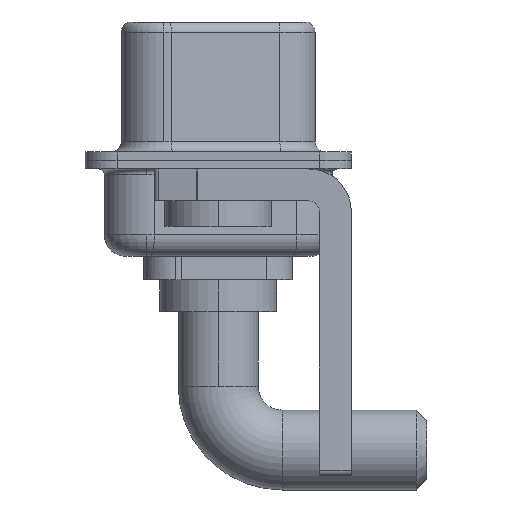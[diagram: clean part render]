
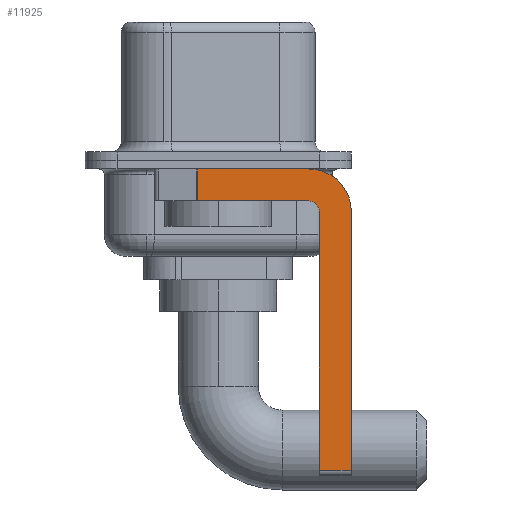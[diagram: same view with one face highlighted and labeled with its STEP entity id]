
A CAD part, left-side view. The second image highlights one B-rep face of the part: STEP entity #11925.
In plain terms, the highlighted planar face has unit normal (-1, 0, 0).
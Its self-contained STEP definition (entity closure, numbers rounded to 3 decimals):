
#54 = LINE ( 'NONE', #5189, #10885 ) ;
#91 = CARTESIAN_POINT ( 'NONE',  ( -2.9, -6.25, -2.4 ) ) ;
#367 = DIRECTION ( 'NONE',  ( 0., -1., 0. ) ) ;
#451 = DIRECTION ( 'NONE',  ( 1., 0., 0. ) ) ;
#596 = VECTOR ( 'NONE', #11595, 1000. ) ;
#710 = VERTEX_POINT ( 'NONE', #9211 ) ;
#754 = VERTEX_POINT ( 'NONE', #5790 ) ;
#1025 = EDGE_CURVE ( 'NONE', #7163, #14038, #7813, .T. ) ;
#1320 = VECTOR ( 'NONE', #367, 1000. ) ;
#1336 = VECTOR ( 'NONE', #6732, 1000. ) ;
#1689 = CARTESIAN_POINT ( 'NONE',  ( -2.9, -4.75, -2.4 ) ) ;
#1849 = ORIENTED_EDGE ( 'NONE', *, *, #5173, .T. ) ;
#1904 = CARTESIAN_POINT ( 'NONE',  ( -2.9, 0.978, -0.4 ) ) ;
#2360 = VECTOR ( 'NONE', #4473, 1000. ) ;
#2472 = EDGE_CURVE ( 'NONE', #4722, #754, #10742, .T. ) ;
#2613 = CARTESIAN_POINT ( 'NONE',  ( -2.9, -4.25, -1.9 ) ) ;
#2647 = CARTESIAN_POINT ( 'NONE',  ( -2.9, 0.978, -1.9 ) ) ;
#2786 = ORIENTED_EDGE ( 'NONE', *, *, #13909, .F. ) ;
#3198 = CARTESIAN_POINT ( 'NONE',  ( -2.9, -4.75, -14.55 ) ) ;
#3556 = CIRCLE ( 'NONE', #6793, 2. ) ;
#3600 = DIRECTION ( 'NONE',  ( -1., 0., 0. ) ) ;
#4473 = DIRECTION ( 'NONE',  ( 0., 0., -1. ) ) ;
#4722 = VERTEX_POINT ( 'NONE', #1904 ) ;
#5173 = EDGE_CURVE ( 'NONE', #16331, #710, #11849, .T. ) ;
#5189 = CARTESIAN_POINT ( 'NONE',  ( -2.9, 3., -0.4 ) ) ;
#5223 = DIRECTION ( 'NONE',  ( 0., 1., 0. ) ) ;
#5396 = LINE ( 'NONE', #6495, #596 ) ;
#5439 = DIRECTION ( 'NONE',  ( 0., 0., -1. ) ) ;
#5602 = EDGE_CURVE ( 'NONE', #6083, #710, #14275, .T. ) ;
#5678 = CARTESIAN_POINT ( 'NONE',  ( -2.9, -4.25, -1.9 ) ) ;
#5790 = CARTESIAN_POINT ( 'NONE',  ( -2.9, 0.978, -1.9 ) ) ;
#6025 = AXIS2_PLACEMENT_3D ( 'NONE', #15941, #13123, #5439 ) ;
#6038 = ORIENTED_EDGE ( 'NONE', *, *, #6094, .F. ) ;
#6083 = VERTEX_POINT ( 'NONE', #91 ) ;
#6094 = EDGE_CURVE ( 'NONE', #14038, #754, #11581, .T. ) ;
#6495 = CARTESIAN_POINT ( 'NONE',  ( -2.9, -4.75, -14.8 ) ) ;
#6732 = DIRECTION ( 'NONE',  ( 0., 0., -1. ) ) ;
#6793 = AXIS2_PLACEMENT_3D ( 'NONE', #11931, #451, #14552 ) ;
#7163 = VERTEX_POINT ( 'NONE', #1689 ) ;
#7592 = ORIENTED_EDGE ( 'NONE', *, *, #8351, .F. ) ;
#7813 = CIRCLE ( 'NONE', #14800, 0.5 ) ;
#8167 = CARTESIAN_POINT ( 'NONE',  ( -2.9, -4.25, -14.55 ) ) ;
#8351 = EDGE_CURVE ( 'NONE', #16331, #7163, #5396, .T. ) ;
#8364 = PLANE ( 'NONE',  #6025 ) ;
#8533 = VERTEX_POINT ( 'NONE', #12171 ) ;
#9000 = EDGE_LOOP ( 'NONE', ( #2786, #15157, #6038, #12072, #7592, #1849, #15802, #12744 ) ) ;
#9030 = CARTESIAN_POINT ( 'NONE',  ( -2.9, -4.25, -2.4 ) ) ;
#9211 = CARTESIAN_POINT ( 'NONE',  ( -2.9, -6.25, -14.55 ) ) ;
#9973 = EDGE_CURVE ( 'NONE', #8533, #6083, #3556, .T. ) ;
#10038 = DIRECTION ( 'NONE',  ( 0., 0., 1. ) ) ;
#10424 = CARTESIAN_POINT ( 'NONE',  ( -2.9, -6.25, -2.4 ) ) ;
#10742 = LINE ( 'NONE', #2647, #2360 ) ;
#10885 = VECTOR ( 'NONE', #15432, 1000. ) ;
#10986 = VECTOR ( 'NONE', #5223, 1000. ) ;
#11581 = LINE ( 'NONE', #2613, #10986 ) ;
#11595 = DIRECTION ( 'NONE',  ( 0., 0., 1. ) ) ;
#11849 = LINE ( 'NONE', #8167, #1320 ) ;
#11925 = ADVANCED_FACE ( 'NONE', ( #14399 ), #8364, .F. ) ;
#11931 = CARTESIAN_POINT ( 'NONE',  ( -2.9, -4.25, -2.4 ) ) ;
#12072 = ORIENTED_EDGE ( 'NONE', *, *, #1025, .F. ) ;
#12171 = CARTESIAN_POINT ( 'NONE',  ( -2.9, -4.25, -0.4 ) ) ;
#12744 = ORIENTED_EDGE ( 'NONE', *, *, #9973, .F. ) ;
#13123 = DIRECTION ( 'NONE',  ( 1., 0., 0. ) ) ;
#13909 = EDGE_CURVE ( 'NONE', #4722, #8533, #54, .T. ) ;
#14038 = VERTEX_POINT ( 'NONE', #5678 ) ;
#14275 = LINE ( 'NONE', #10424, #1336 ) ;
#14399 = FACE_OUTER_BOUND ( 'NONE', #9000, .T. ) ;
#14552 = DIRECTION ( 'NONE',  ( 0., 0., -1. ) ) ;
#14800 = AXIS2_PLACEMENT_3D ( 'NONE', #9030, #3600, #10038 ) ;
#15157 = ORIENTED_EDGE ( 'NONE', *, *, #2472, .T. ) ;
#15432 = DIRECTION ( 'NONE',  ( 0., -1., 0. ) ) ;
#15802 = ORIENTED_EDGE ( 'NONE', *, *, #5602, .F. ) ;
#15941 = CARTESIAN_POINT ( 'NONE',  ( -2.9, -4.25, -2.4 ) ) ;
#16331 = VERTEX_POINT ( 'NONE', #3198 ) ;
